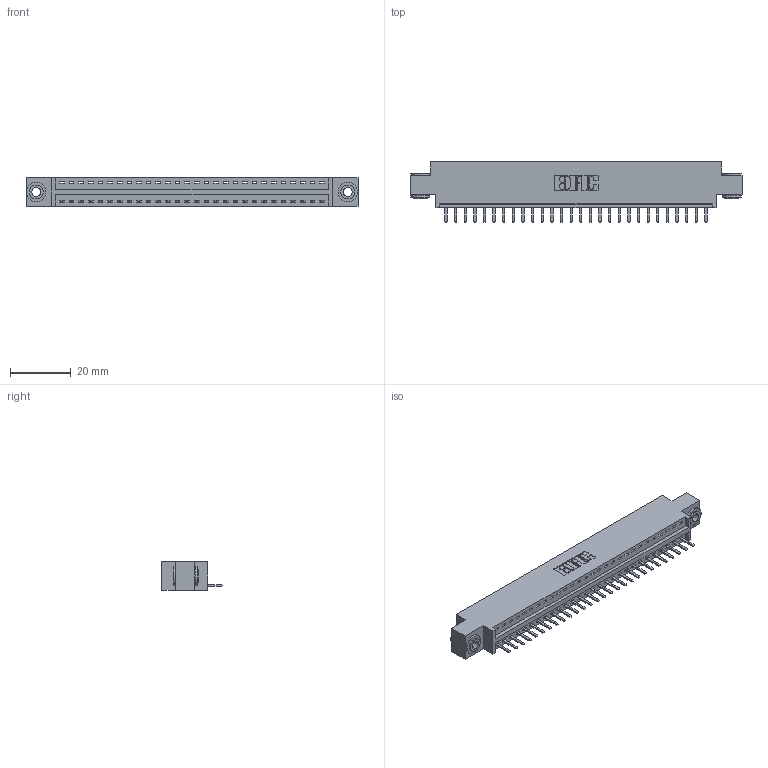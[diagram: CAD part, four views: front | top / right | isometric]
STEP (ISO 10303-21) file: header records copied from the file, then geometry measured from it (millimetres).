
FILE_DESCRIPTION (( 'STEP AP203' ), '1' );
FILE_NAME ('396-028-520-603.STEP', '2018-09-05T02:28:50', ( '' ), ( '' ), 'SwSTEP 2.0', 'SolidWorks 2016', '' );
FILE_SCHEMA (( 'CONFIG_CONTROL_DESIGN' ));
Length unit declared in the file: inch
Products named in the file (4): 346 Part_0.170 Offset - 0.156 Dia-TH; 345-292-001_345-293-120; 345-250-002_345-250-002-102; 396-028-520-603
Assembly tree (31 placements, depth 2):
  396-028-520-603
    346 Part_0.170 Offset - 0.156 Dia-TH
    345-292-001_345-293-120  x28
    345-250-002_345-250-002-102  x2
Bounding box: 109.47 x 20.02 x 9.4 mm (x, y, z)
Volume: 10166.9 mm3; surface area: 12666.8 mm2
Topology: 31 solids, 31 shells, 1900 faces, 5569 edges, 3634 vertices
Faces by surface type: plane 1266, cylinder 626, cone 8
Entity records: 20158 total; most frequent: CARTESIAN_POINT 3451, ORIENTED_EDGE 3394, DIRECTION 3079, EDGE_CURVE 1697, LINE 1425, VECTOR 1425, VERTEX_POINT 1126, AXIS2_PLACEMENT_3D 827
